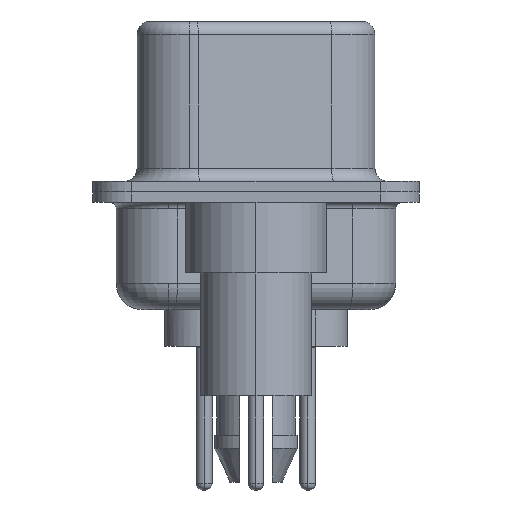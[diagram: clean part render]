
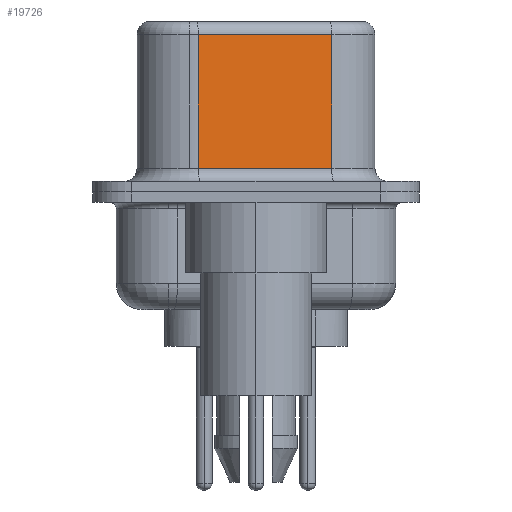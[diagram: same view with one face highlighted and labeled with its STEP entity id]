
A CAD part, left-side view. The second image highlights one B-rep face of the part: STEP entity #19726.
In plain terms, the highlighted planar face has unit normal (-0.985, -0.174, 0).
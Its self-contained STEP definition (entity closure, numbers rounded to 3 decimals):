
#171 = VERTEX_POINT ( 'NONE', #472 ) ;
#342 = DIRECTION ( 'NONE',  ( -0.174, 0.985, 0. ) ) ;
#472 = CARTESIAN_POINT ( 'NONE',  ( 4.555, -2.897, 0.9 ) ) ;
#1936 = EDGE_CURVE ( 'NONE', #8499, #20411, #19990, .T. ) ;
#2500 = LINE ( 'NONE', #11244, #19723 ) ;
#2748 = CARTESIAN_POINT ( 'NONE',  ( 3.655, 2.203, 6.52 ) ) ;
#3078 = ORIENTED_EDGE ( 'NONE', *, *, #9163, .T. ) ;
#3667 = CARTESIAN_POINT ( 'NONE',  ( 4.555, -2.897, 6.02 ) ) ;
#3941 = DIRECTION ( 'NONE',  ( 0.985, 0.174, 0. ) ) ;
#4675 = DIRECTION ( 'NONE',  ( 0., 0., -1. ) ) ;
#4822 = EDGE_LOOP ( 'NONE', ( #16049, #7496, #14020, #3078 ) ) ;
#5275 = VECTOR ( 'NONE', #342, 1000. ) ;
#5898 = CARTESIAN_POINT ( 'NONE',  ( 3.655, 2.203, 0.9 ) ) ;
#7496 = ORIENTED_EDGE ( 'NONE', *, *, #14681, .T. ) ;
#8063 = CARTESIAN_POINT ( 'NONE',  ( 3.655, 2.203, 6.02 ) ) ;
#8499 = VERTEX_POINT ( 'NONE', #8063 ) ;
#9163 = EDGE_CURVE ( 'NONE', #20411, #171, #2500, .T. ) ;
#10590 = CARTESIAN_POINT ( 'NONE',  ( 4.555, -2.897, 6.52 ) ) ;
#10870 = VECTOR ( 'NONE', #20080, 1000. ) ;
#11244 = CARTESIAN_POINT ( 'NONE',  ( 4.555, -2.897, 0.9 ) ) ;
#11399 = LINE ( 'NONE', #13408, #10870 ) ;
#11676 = FACE_OUTER_BOUND ( 'NONE', #4822, .T. ) ;
#11875 = EDGE_CURVE ( 'NONE', #12451, #171, #11399, .T. ) ;
#12451 = VERTEX_POINT ( 'NONE', #21402 ) ;
#13408 = CARTESIAN_POINT ( 'NONE',  ( 4.555, -2.897, 6.52 ) ) ;
#13956 = PLANE ( 'NONE',  #16627 ) ;
#14020 = ORIENTED_EDGE ( 'NONE', *, *, #1936, .T. ) ;
#14681 = EDGE_CURVE ( 'NONE', #12451, #8499, #14700, .T. ) ;
#14700 = LINE ( 'NONE', #3667, #5275 ) ;
#15603 = VECTOR ( 'NONE', #4675, 1000. ) ;
#15617 = DIRECTION ( 'NONE',  ( -0.174, 0.985, 0. ) ) ;
#16049 = ORIENTED_EDGE ( 'NONE', *, *, #11875, .F. ) ;
#16260 = DIRECTION ( 'NONE',  ( 0.174, -0.985, 0. ) ) ;
#16627 = AXIS2_PLACEMENT_3D ( 'NONE', #10590, #3941, #15617 ) ;
#19723 = VECTOR ( 'NONE', #16260, 1000. ) ;
#19726 = ADVANCED_FACE ( 'NONE', ( #11676 ), #13956, .F. ) ;
#19990 = LINE ( 'NONE', #2748, #15603 ) ;
#20080 = DIRECTION ( 'NONE',  ( 0., 0., -1. ) ) ;
#20411 = VERTEX_POINT ( 'NONE', #5898 ) ;
#21402 = CARTESIAN_POINT ( 'NONE',  ( 4.555, -2.897, 6.02 ) ) ;
